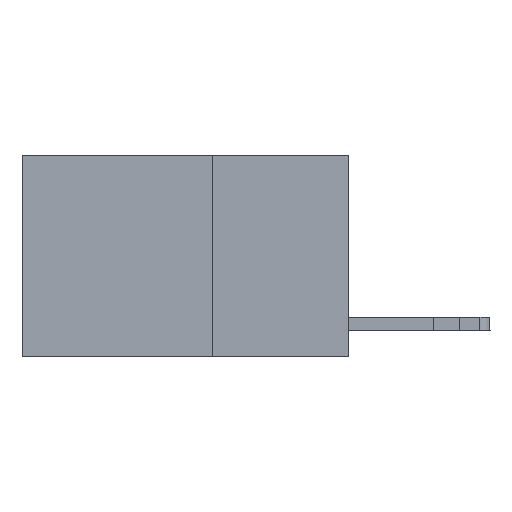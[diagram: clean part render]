
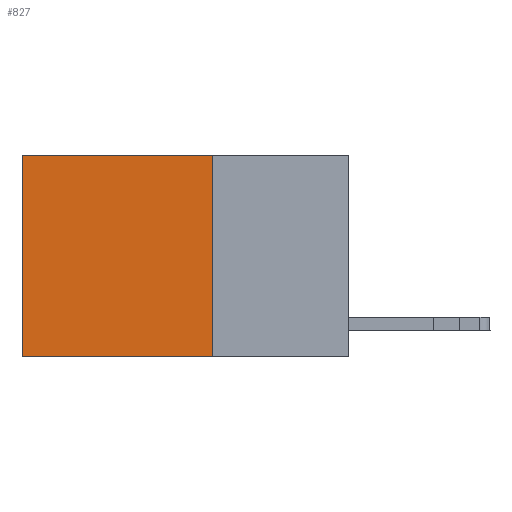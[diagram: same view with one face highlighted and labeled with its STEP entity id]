
A CAD part, left-side view. The second image highlights one B-rep face of the part: STEP entity #827.
In plain terms, the highlighted planar face has unit normal (-1, 0, 0).
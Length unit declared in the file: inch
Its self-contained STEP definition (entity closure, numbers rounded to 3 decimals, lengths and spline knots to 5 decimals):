
#130 = DIRECTION ( 'NONE',  ( 0., 1., 0. ) ) ;
#827 = ADVANCED_FACE ( 'NONE', ( #13498 ), #11586, .F. ) ;
#914 = CARTESIAN_POINT ( 'NONE',  ( 0.2625, 0.6, 0. ) ) ;
#1259 = DIRECTION ( 'NONE',  ( 0., 1., 0. ) ) ;
#1394 = ORIENTED_EDGE ( 'NONE', *, *, #14540, .T. ) ;
#3276 = LINE ( 'NONE', #13426, #4456 ) ;
#3432 = VERTEX_POINT ( 'NONE', #914 ) ;
#3540 = LINE ( 'NONE', #6237, #9104 ) ;
#3836 = CARTESIAN_POINT ( 'NONE',  ( 0.2625, 0.25, -0.37 ) ) ;
#4361 = EDGE_CURVE ( 'NONE', #6780, #12284, #3276, .T. ) ;
#4456 = VECTOR ( 'NONE', #13386, 39.37008 ) ;
#4813 = ORIENTED_EDGE ( 'NONE', *, *, #8599, .T. ) ;
#4829 = VECTOR ( 'NONE', #1259, 39.37008 ) ;
#6237 = CARTESIAN_POINT ( 'NONE',  ( 0.2625, 0.25, -0.37 ) ) ;
#6313 = DIRECTION ( 'NONE',  ( 0., 0., -1. ) ) ;
#6780 = VERTEX_POINT ( 'NONE', #10278 ) ;
#7090 = EDGE_CURVE ( 'NONE', #12284, #7179, #3540, .T. ) ;
#7179 = VERTEX_POINT ( 'NONE', #10919 ) ;
#8599 = EDGE_CURVE ( 'NONE', #6780, #3432, #13760, .T. ) ;
#8633 = CARTESIAN_POINT ( 'NONE',  ( 0.2625, 0.6, 0. ) ) ;
#9104 = VECTOR ( 'NONE', #130, 39.37008 ) ;
#10278 = CARTESIAN_POINT ( 'NONE',  ( 0.2625, 0.25, 0. ) ) ;
#10306 = EDGE_LOOP ( 'NONE', ( #1394, #11095, #13374, #4813 ) ) ;
#10552 = AXIS2_PLACEMENT_3D ( 'NONE', #11623, #11369, #11291 ) ;
#10680 = VECTOR ( 'NONE', #6313, 39.37008 ) ;
#10919 = CARTESIAN_POINT ( 'NONE',  ( 0.2625, 0.6, -0.37 ) ) ;
#11042 = LINE ( 'NONE', #8633, #10680 ) ;
#11095 = ORIENTED_EDGE ( 'NONE', *, *, #7090, .F. ) ;
#11291 = DIRECTION ( 'NONE',  ( 0., 0., -1. ) ) ;
#11369 = DIRECTION ( 'NONE',  ( 1., 0., 0. ) ) ;
#11586 = PLANE ( 'NONE',  #10552 ) ;
#11623 = CARTESIAN_POINT ( 'NONE',  ( 0.2625, 0.25, 0. ) ) ;
#12284 = VERTEX_POINT ( 'NONE', #3836 ) ;
#13374 = ORIENTED_EDGE ( 'NONE', *, *, #4361, .F. ) ;
#13386 = DIRECTION ( 'NONE',  ( 0., 0., -1. ) ) ;
#13426 = CARTESIAN_POINT ( 'NONE',  ( 0.2625, 0.25, 0. ) ) ;
#13498 = FACE_OUTER_BOUND ( 'NONE', #10306, .T. ) ;
#13760 = LINE ( 'NONE', #14823, #4829 ) ;
#14540 = EDGE_CURVE ( 'NONE', #3432, #7179, #11042, .T. ) ;
#14823 = CARTESIAN_POINT ( 'NONE',  ( 0.2625, 0.25, 0. ) ) ;
